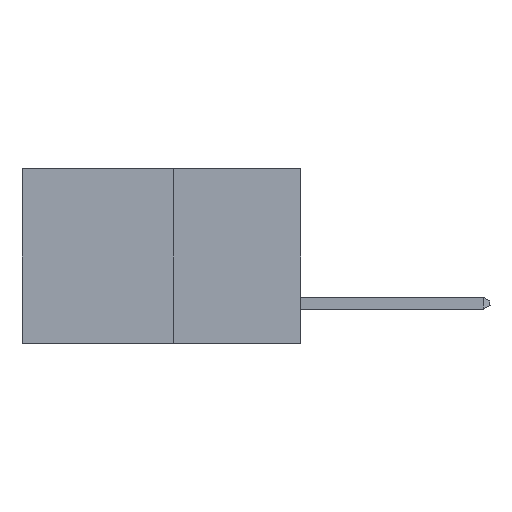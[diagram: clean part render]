
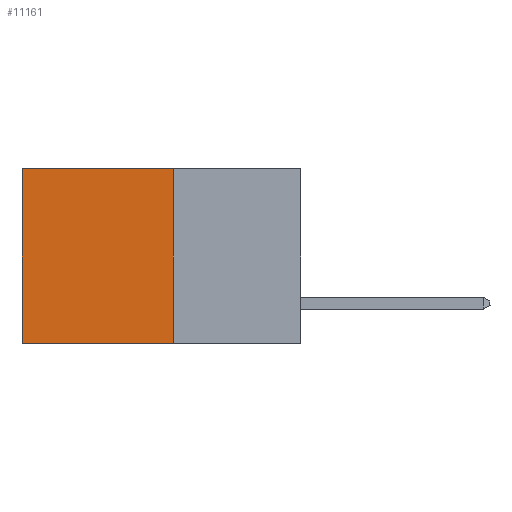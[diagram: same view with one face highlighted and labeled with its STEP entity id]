
A CAD part, left-side view. The second image highlights one B-rep face of the part: STEP entity #11161.
In plain terms, the highlighted planar face has unit normal (-1, 0, 0).
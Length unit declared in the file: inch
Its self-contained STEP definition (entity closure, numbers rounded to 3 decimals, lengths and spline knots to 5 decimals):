
#755 = DIRECTION ( 'NONE',  ( 0., 1., 0. ) ) ;
#1785 = CARTESIAN_POINT ( 'NONE',  ( 0.277, 0.27, 0. ) ) ;
#2109 = DIRECTION ( 'NONE',  ( 0., 0., -1. ) ) ;
#5112 = DIRECTION ( 'NONE',  ( 0., 0., -1. ) ) ;
#5138 = VERTEX_POINT ( 'NONE', #21353 ) ;
#5328 = ORIENTED_EDGE ( 'NONE', *, *, #10923, .F. ) ;
#6584 = LINE ( 'NONE', #16855, #17088 ) ;
#7010 = EDGE_LOOP ( 'NONE', ( #16307, #25548, #5328, #9610 ) ) ;
#7487 = EDGE_CURVE ( 'NONE', #13709, #5138, #10521, .T. ) ;
#8241 = PLANE ( 'NONE',  #23471 ) ;
#8957 = EDGE_CURVE ( 'NONE', #24646, #21321, #10754, .T. ) ;
#9610 = ORIENTED_EDGE ( 'NONE', *, *, #8957, .T. ) ;
#10521 = LINE ( 'NONE', #19588, #20962 ) ;
#10754 = LINE ( 'NONE', #17601, #16342 ) ;
#10923 = EDGE_CURVE ( 'NONE', #24646, #13709, #18213, .T. ) ;
#11161 = ADVANCED_FACE ( 'NONE', ( #24762 ), #8241, .F. ) ;
#12479 = DIRECTION ( 'NONE',  ( 1., 0., 0. ) ) ;
#12688 = VECTOR ( 'NONE', #5112, 39.37008 ) ;
#13709 = VERTEX_POINT ( 'NONE', #24339 ) ;
#15581 = CARTESIAN_POINT ( 'NONE',  ( 0.277, 0.27, -0.37 ) ) ;
#16307 = ORIENTED_EDGE ( 'NONE', *, *, #22128, .T. ) ;
#16342 = VECTOR ( 'NONE', #755, 39.37008 ) ;
#16592 = CARTESIAN_POINT ( 'NONE',  ( 0.277, 0.27, -0.37 ) ) ;
#16855 = CARTESIAN_POINT ( 'NONE',  ( 0.277, 0.59, -0.37 ) ) ;
#17088 = VECTOR ( 'NONE', #2109, 39.37008 ) ;
#17601 = CARTESIAN_POINT ( 'NONE',  ( 0.277, 0.27, 0. ) ) ;
#18213 = LINE ( 'NONE', #15581, #12688 ) ;
#19524 = DIRECTION ( 'NONE',  ( 0., 1., 0. ) ) ;
#19588 = CARTESIAN_POINT ( 'NONE',  ( 0.277, 0.27, -0.37 ) ) ;
#20962 = VECTOR ( 'NONE', #19524, 39.37008 ) ;
#21321 = VERTEX_POINT ( 'NONE', #22714 ) ;
#21353 = CARTESIAN_POINT ( 'NONE',  ( 0.277, 0.59, -0.37 ) ) ;
#22128 = EDGE_CURVE ( 'NONE', #21321, #5138, #6584, .T. ) ;
#22714 = CARTESIAN_POINT ( 'NONE',  ( 0.277, 0.59, 0. ) ) ;
#23471 = AXIS2_PLACEMENT_3D ( 'NONE', #16592, #12479, #27042 ) ;
#24339 = CARTESIAN_POINT ( 'NONE',  ( 0.277, 0.27, -0.37 ) ) ;
#24646 = VERTEX_POINT ( 'NONE', #1785 ) ;
#24762 = FACE_OUTER_BOUND ( 'NONE', #7010, .T. ) ;
#25548 = ORIENTED_EDGE ( 'NONE', *, *, #7487, .F. ) ;
#27042 = DIRECTION ( 'NONE',  ( 0., 0., -1. ) ) ;
